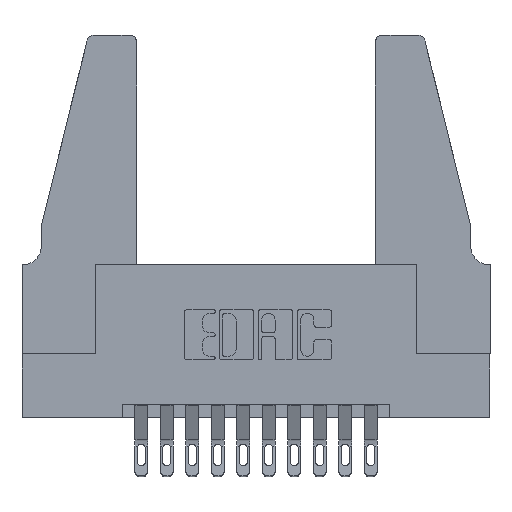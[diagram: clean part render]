
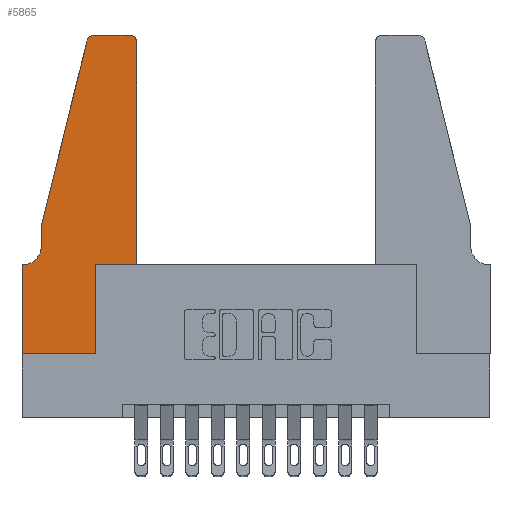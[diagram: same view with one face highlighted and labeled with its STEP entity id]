
A CAD part, top view. The second image highlights one B-rep face of the part: STEP entity #5865.
In plain terms, the highlighted planar face has unit normal (0, 0, 1).
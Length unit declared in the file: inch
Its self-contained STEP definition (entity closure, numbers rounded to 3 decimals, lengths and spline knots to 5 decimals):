
#41 = CIRCLE ( 'NONE', #10345, 0.07 ) ;
#42 = VERTEX_POINT ( 'NONE', #4246 ) ;
#250 = CIRCLE ( 'NONE', #11856, 0.03 ) ;
#581 = VERTEX_POINT ( 'NONE', #2861 ) ;
#687 = VECTOR ( 'NONE', #1885, 39.37008 ) ;
#696 = VECTOR ( 'NONE', #12431, 39.37008 ) ;
#877 = LINE ( 'NONE', #1431, #687 ) ;
#992 = CARTESIAN_POINT ( 'NONE',  ( 0.2865, 0.35, 0.37 ) ) ;
#1031 = CARTESIAN_POINT ( 'NONE',  ( 0.0755, 0.5, 0.37 ) ) ;
#1034 = VECTOR ( 'NONE', #10142, 39.37008 ) ;
#1431 = CARTESIAN_POINT ( 'NONE',  ( 0.4505, 0.35, 0.37 ) ) ;
#1750 = VERTEX_POINT ( 'NONE', #9928 ) ;
#1790 = DIRECTION ( 'NONE',  ( 0., -1., 0. ) ) ;
#1885 = DIRECTION ( 'NONE',  ( 1., 0., 0. ) ) ;
#1927 = VECTOR ( 'NONE', #6436, 39.37008 ) ;
#2106 = DIRECTION ( 'NONE',  ( 0., 0., 1. ) ) ;
#2255 = EDGE_CURVE ( 'NONE', #12189, #581, #14233, .T. ) ;
#2402 = ORIENTED_EDGE ( 'NONE', *, *, #4972, .T. ) ;
#2797 = CARTESIAN_POINT ( 'NONE',  ( 0.25487, 1.22718, 0.37 ) ) ;
#2861 = CARTESIAN_POINT ( 'NONE',  ( 0.0755, 0.42, 0.37 ) ) ;
#2987 = ORIENTED_EDGE ( 'NONE', *, *, #11151, .T. ) ;
#3319 = DIRECTION ( 'NONE',  ( 1., 0., 0. ) ) ;
#3389 = DIRECTION ( 'NONE',  ( 1., 0., 0. ) ) ;
#3469 = CARTESIAN_POINT ( 'NONE',  ( 0., 0.35, 0.37 ) ) ;
#3535 = FACE_OUTER_BOUND ( 'NONE', #6992, .T. ) ;
#3818 = ORIENTED_EDGE ( 'NONE', *, *, #14346, .T. ) ;
#3879 = LINE ( 'NONE', #12219, #1927 ) ;
#4051 = LINE ( 'NONE', #9080, #1034 ) ;
#4246 = CARTESIAN_POINT ( 'NONE',  ( 0., 0., 0.37 ) ) ;
#4850 = CARTESIAN_POINT ( 'NONE',  ( 0., 0., 0.37 ) ) ;
#4972 = EDGE_CURVE ( 'NONE', #1750, #11720, #11497, .T. ) ;
#4993 = AXIS2_PLACEMENT_3D ( 'NONE', #3469, #8940, #3319 ) ;
#5047 = CARTESIAN_POINT ( 'NONE',  ( 0.0055, 0.35, 0.37 ) ) ;
#5179 = VERTEX_POINT ( 'NONE', #14008 ) ;
#5192 = VECTOR ( 'NONE', #9653, 39.37008 ) ;
#5212 = ORIENTED_EDGE ( 'NONE', *, *, #12491, .T. ) ;
#5278 = CARTESIAN_POINT ( 'NONE',  ( 0., 0.35, 0.37 ) ) ;
#5824 = ORIENTED_EDGE ( 'NONE', *, *, #7702, .T. ) ;
#5854 = CARTESIAN_POINT ( 'NONE',  ( 0.2605, 1.25, 0.37 ) ) ;
#5865 = ADVANCED_FACE ( 'NONE', ( #3535 ), #7807, .T. ) ;
#6113 = EDGE_CURVE ( 'NONE', #9646, #12189, #4051, .T. ) ;
#6265 = CARTESIAN_POINT ( 'NONE',  ( 0.4505, 0.35, 0.37 ) ) ;
#6331 = ORIENTED_EDGE ( 'NONE', *, *, #9300, .T. ) ;
#6436 = DIRECTION ( 'NONE',  ( -1., 0., 0. ) ) ;
#6626 = VERTEX_POINT ( 'NONE', #13405 ) ;
#6992 = EDGE_LOOP ( 'NONE', ( #12956, #2987, #13072, #12525, #5212, #6331, #3818, #10353, #2402, #5824, #9776, #10230 ) ) ;
#7036 = DIRECTION ( 'NONE',  ( -1., 0., 0. ) ) ;
#7386 = CARTESIAN_POINT ( 'NONE',  ( 0.0755, 0.5, 0.37 ) ) ;
#7508 = CARTESIAN_POINT ( 'NONE',  ( 0.0055, 0.42, 0.37 ) ) ;
#7599 = DIRECTION ( 'NONE',  ( -1., 0., 0. ) ) ;
#7702 = EDGE_CURVE ( 'NONE', #11720, #6626, #877, .T. ) ;
#7807 = PLANE ( 'NONE',  #4993 ) ;
#8042 = VECTOR ( 'NONE', #10062, 39.37008 ) ;
#8553 = VECTOR ( 'NONE', #13805, 39.37008 ) ;
#8620 = LINE ( 'NONE', #5854, #13744 ) ;
#8868 = CARTESIAN_POINT ( 'NONE',  ( 0.284, 1.22, 0.37 ) ) ;
#8940 = DIRECTION ( 'NONE',  ( 0., 0., 1. ) ) ;
#9080 = CARTESIAN_POINT ( 'NONE',  ( 0.0755, 0.5, 0.37 ) ) ;
#9218 = VERTEX_POINT ( 'NONE', #14492 ) ;
#9300 = EDGE_CURVE ( 'NONE', #11372, #14164, #3879, .T. ) ;
#9451 = LINE ( 'NONE', #11142, #8042 ) ;
#9531 = VERTEX_POINT ( 'NONE', #11420 ) ;
#9646 = VERTEX_POINT ( 'NONE', #2797 ) ;
#9653 = DIRECTION ( 'NONE',  ( 0., 1., 0. ) ) ;
#9776 = ORIENTED_EDGE ( 'NONE', *, *, #12507, .T. ) ;
#9797 = CIRCLE ( 'NONE', #11345, 0.03 ) ;
#9928 = CARTESIAN_POINT ( 'NONE',  ( 0.2865, 0., 0.37 ) ) ;
#10061 = EDGE_CURVE ( 'NONE', #5179, #9218, #8620, .T. ) ;
#10062 = DIRECTION ( 'NONE',  ( 1., 0., 0. ) ) ;
#10131 = LINE ( 'NONE', #6265, #5192 ) ;
#10142 = DIRECTION ( 'NONE',  ( -0.239, -0.971, 0. ) ) ;
#10230 = ORIENTED_EDGE ( 'NONE', *, *, #13221, .T. ) ;
#10345 = AXIS2_PLACEMENT_3D ( 'NONE', #7508, #11042, #7599 ) ;
#10353 = ORIENTED_EDGE ( 'NONE', *, *, #11683, .T. ) ;
#10536 = VECTOR ( 'NONE', #1790, 39.37008 ) ;
#10641 = DIRECTION ( 'NONE',  ( 0., 0., 1. ) ) ;
#11042 = DIRECTION ( 'NONE',  ( 0., 0., -1. ) ) ;
#11142 = CARTESIAN_POINT ( 'NONE',  ( 0., 0., 0.37 ) ) ;
#11151 = EDGE_CURVE ( 'NONE', #9218, #9646, #9797, .T. ) ;
#11193 = LINE ( 'NONE', #4850, #8553 ) ;
#11345 = AXIS2_PLACEMENT_3D ( 'NONE', #8868, #2106, #3389 ) ;
#11372 = VERTEX_POINT ( 'NONE', #5047 ) ;
#11377 = CARTESIAN_POINT ( 'NONE',  ( 0.2865, 0.35, 0.37 ) ) ;
#11420 = CARTESIAN_POINT ( 'NONE',  ( 0.4505, 1.22, 0.37 ) ) ;
#11497 = LINE ( 'NONE', #11377, #696 ) ;
#11678 = DIRECTION ( 'NONE',  ( 1., 0., 0. ) ) ;
#11683 = EDGE_CURVE ( 'NONE', #42, #1750, #9451, .T. ) ;
#11720 = VERTEX_POINT ( 'NONE', #992 ) ;
#11856 = AXIS2_PLACEMENT_3D ( 'NONE', #13850, #10641, #11678 ) ;
#12189 = VERTEX_POINT ( 'NONE', #1031 ) ;
#12219 = CARTESIAN_POINT ( 'NONE',  ( 0.0755, 0.35, 0.37 ) ) ;
#12431 = DIRECTION ( 'NONE',  ( 0., 1., 0. ) ) ;
#12491 = EDGE_CURVE ( 'NONE', #581, #11372, #41, .T. ) ;
#12507 = EDGE_CURVE ( 'NONE', #6626, #9531, #10131, .T. ) ;
#12525 = ORIENTED_EDGE ( 'NONE', *, *, #2255, .T. ) ;
#12956 = ORIENTED_EDGE ( 'NONE', *, *, #10061, .T. ) ;
#13072 = ORIENTED_EDGE ( 'NONE', *, *, #6113, .T. ) ;
#13221 = EDGE_CURVE ( 'NONE', #9531, #5179, #250, .T. ) ;
#13405 = CARTESIAN_POINT ( 'NONE',  ( 0.4505, 0.35, 0.37 ) ) ;
#13744 = VECTOR ( 'NONE', #7036, 39.37008 ) ;
#13805 = DIRECTION ( 'NONE',  ( 0., -1., 0. ) ) ;
#13850 = CARTESIAN_POINT ( 'NONE',  ( 0.4205, 1.22, 0.37 ) ) ;
#14008 = CARTESIAN_POINT ( 'NONE',  ( 0.4205, 1.25, 0.37 ) ) ;
#14164 = VERTEX_POINT ( 'NONE', #5278 ) ;
#14233 = LINE ( 'NONE', #7386, #10536 ) ;
#14346 = EDGE_CURVE ( 'NONE', #14164, #42, #11193, .T. ) ;
#14492 = CARTESIAN_POINT ( 'NONE',  ( 0.284, 1.25, 0.37 ) ) ;
